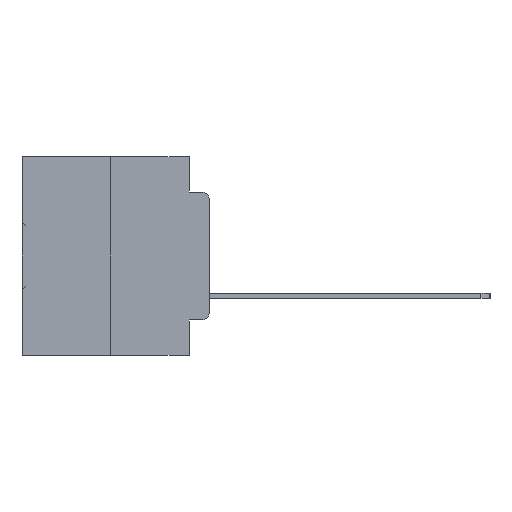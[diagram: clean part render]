
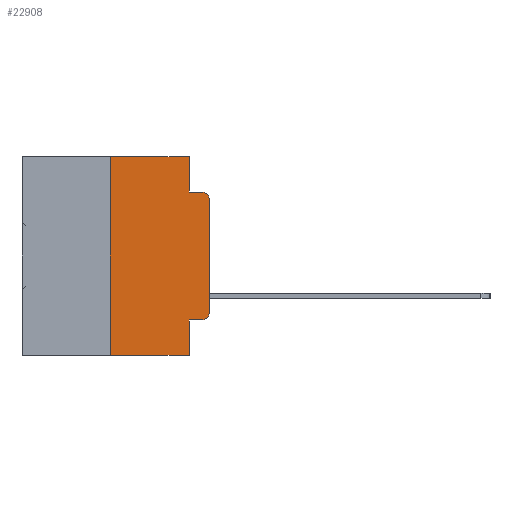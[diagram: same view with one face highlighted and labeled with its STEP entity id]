
A CAD part, left-side view. The second image highlights one B-rep face of the part: STEP entity #22908.
In plain terms, the highlighted planar face has unit normal (-1, 0, 0).
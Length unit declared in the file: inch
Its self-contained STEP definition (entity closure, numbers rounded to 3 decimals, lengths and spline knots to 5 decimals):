
#1056 = VECTOR ( 'NONE', #15404, 39.37008 ) ;
#1269 = CARTESIAN_POINT ( 'NONE',  ( 0., 0.051, -0.4115 ) ) ;
#1738 = ORIENTED_EDGE ( 'NONE', *, *, #35972, .T. ) ;
#2229 = ORIENTED_EDGE ( 'NONE', *, *, #19711, .F. ) ;
#2500 = DIRECTION ( 'NONE',  ( -1., 0., 0. ) ) ;
#3586 = CARTESIAN_POINT ( 'NONE',  ( 0., 0.25, -0.5 ) ) ;
#3743 = CARTESIAN_POINT ( 'NONE',  ( 0., 0.051, -0.4115 ) ) ;
#4054 = ORIENTED_EDGE ( 'NONE', *, *, #25440, .T. ) ;
#4241 = VECTOR ( 'NONE', #36297, 39.37008 ) ;
#4340 = VERTEX_POINT ( 'NONE', #30732 ) ;
#5243 = DIRECTION ( 'NONE',  ( 0., 0., -1. ) ) ;
#6064 = LINE ( 'NONE', #13987, #4241 ) ;
#6784 = CARTESIAN_POINT ( 'NONE',  ( 0., 0.02, -0.1085 ) ) ;
#7334 = VERTEX_POINT ( 'NONE', #12766 ) ;
#7928 = CARTESIAN_POINT ( 'NONE',  ( 0., 0.02, -0.4115 ) ) ;
#8266 = EDGE_LOOP ( 'NONE', ( #1738, #24762, #33824, #27350, #21691, #29962, #24350, #2229, #26063, #4054 ) ) ;
#8733 = LINE ( 'NONE', #10281, #33962 ) ;
#9096 = EDGE_CURVE ( 'NONE', #15135, #34101, #36450, .T. ) ;
#9732 = DIRECTION ( 'NONE',  ( 0., 0., -1. ) ) ;
#9747 = VECTOR ( 'NONE', #12873, 39.37008 ) ;
#9796 = VERTEX_POINT ( 'NONE', #31091 ) ;
#10281 = CARTESIAN_POINT ( 'NONE',  ( 0., 0.25, 0. ) ) ;
#10906 = DIRECTION ( 'NONE',  ( 1., 0., 0. ) ) ;
#11602 = DIRECTION ( 'NONE',  ( 0., -1., 0. ) ) ;
#11873 = CIRCLE ( 'NONE', #14674, 0.02 ) ;
#11953 = EDGE_CURVE ( 'NONE', #4340, #20574, #22420, .T. ) ;
#12243 = LINE ( 'NONE', #31392, #19895 ) ;
#12766 = CARTESIAN_POINT ( 'NONE',  ( 0., 0., -0.3915 ) ) ;
#12873 = DIRECTION ( 'NONE',  ( 0., -1., 0. ) ) ;
#13215 = DIRECTION ( 'NONE',  ( 0., 0., 1. ) ) ;
#13987 = CARTESIAN_POINT ( 'NONE',  ( 0., 0.473, 0. ) ) ;
#14126 = CARTESIAN_POINT ( 'NONE',  ( 0., 0.25, 0. ) ) ;
#14674 = AXIS2_PLACEMENT_3D ( 'NONE', #19851, #2500, #22746 ) ;
#15135 = VERTEX_POINT ( 'NONE', #1269 ) ;
#15404 = DIRECTION ( 'NONE',  ( 0., 0., 1. ) ) ;
#15636 = LINE ( 'NONE', #27138, #16526 ) ;
#16012 = DIRECTION ( 'NONE',  ( 0., 0., -1. ) ) ;
#16526 = VECTOR ( 'NONE', #16012, 39.37008 ) ;
#17277 = FACE_OUTER_BOUND ( 'NONE', #8266, .T. ) ;
#19446 = CARTESIAN_POINT ( 'NONE',  ( 0., 0.473, 0. ) ) ;
#19663 = EDGE_CURVE ( 'NONE', #9796, #20574, #32316, .T. ) ;
#19711 = EDGE_CURVE ( 'NONE', #15135, #25447, #15636, .T. ) ;
#19851 = CARTESIAN_POINT ( 'NONE',  ( 0., 0.02, -0.3915 ) ) ;
#19895 = VECTOR ( 'NONE', #11602, 39.37008 ) ;
#19955 = VECTOR ( 'NONE', #5243, 39.37008 ) ;
#20574 = VERTEX_POINT ( 'NONE', #32789 ) ;
#21527 = CARTESIAN_POINT ( 'NONE',  ( 0., 0.051, -0.0885 ) ) ;
#21691 = ORIENTED_EDGE ( 'NONE', *, *, #28326, .F. ) ;
#21794 = AXIS2_PLACEMENT_3D ( 'NONE', #6784, #26805, #9732 ) ;
#22075 = EDGE_CURVE ( 'NONE', #27479, #34710, #8733, .T. ) ;
#22420 = CIRCLE ( 'NONE', #21794, 0.02 ) ;
#22571 = CARTESIAN_POINT ( 'NONE',  ( 0., 0.051, 0. ) ) ;
#22730 = VERTEX_POINT ( 'NONE', #32839 ) ;
#22746 = DIRECTION ( 'NONE',  ( 0., 0., -1. ) ) ;
#22908 = ADVANCED_FACE ( 'NONE', ( #17277 ), #36146, .F. ) ;
#23246 = LINE ( 'NONE', #32216, #1056 ) ;
#23711 = EDGE_CURVE ( 'NONE', #27479, #25447, #12243, .T. ) ;
#24350 = ORIENTED_EDGE ( 'NONE', *, *, #23711, .T. ) ;
#24762 = ORIENTED_EDGE ( 'NONE', *, *, #11953, .T. ) ;
#25440 = EDGE_CURVE ( 'NONE', #34101, #7334, #11873, .T. ) ;
#25447 = VERTEX_POINT ( 'NONE', #30992 ) ;
#26063 = ORIENTED_EDGE ( 'NONE', *, *, #9096, .T. ) ;
#26800 = DIRECTION ( 'NONE',  ( 0., -1., 0. ) ) ;
#26805 = DIRECTION ( 'NONE',  ( -1., 0., 0. ) ) ;
#27138 = CARTESIAN_POINT ( 'NONE',  ( 0., 0.051, 0. ) ) ;
#27350 = ORIENTED_EDGE ( 'NONE', *, *, #30926, .F. ) ;
#27398 = LINE ( 'NONE', #22571, #19955 ) ;
#27479 = VERTEX_POINT ( 'NONE', #3586 ) ;
#28326 = EDGE_CURVE ( 'NONE', #34710, #22730, #6064, .T. ) ;
#28570 = AXIS2_PLACEMENT_3D ( 'NONE', #19446, #10906, #30699 ) ;
#29089 = VECTOR ( 'NONE', #26800, 39.37008 ) ;
#29962 = ORIENTED_EDGE ( 'NONE', *, *, #22075, .F. ) ;
#30699 = DIRECTION ( 'NONE',  ( 0., 0., -1. ) ) ;
#30732 = CARTESIAN_POINT ( 'NONE',  ( 0., 0., -0.1085 ) ) ;
#30926 = EDGE_CURVE ( 'NONE', #22730, #9796, #27398, .T. ) ;
#30992 = CARTESIAN_POINT ( 'NONE',  ( 0., 0.051, -0.5 ) ) ;
#31091 = CARTESIAN_POINT ( 'NONE',  ( 0., 0.051, -0.0885 ) ) ;
#31392 = CARTESIAN_POINT ( 'NONE',  ( 0., 0.473, -0.5 ) ) ;
#32216 = CARTESIAN_POINT ( 'NONE',  ( 0., 0., 0. ) ) ;
#32316 = LINE ( 'NONE', #21527, #9747 ) ;
#32789 = CARTESIAN_POINT ( 'NONE',  ( 0., 0.02, -0.0885 ) ) ;
#32839 = CARTESIAN_POINT ( 'NONE',  ( 0., 0.051, 0. ) ) ;
#33824 = ORIENTED_EDGE ( 'NONE', *, *, #19663, .F. ) ;
#33962 = VECTOR ( 'NONE', #13215, 39.37008 ) ;
#34101 = VERTEX_POINT ( 'NONE', #7928 ) ;
#34710 = VERTEX_POINT ( 'NONE', #14126 ) ;
#35972 = EDGE_CURVE ( 'NONE', #7334, #4340, #23246, .T. ) ;
#36146 = PLANE ( 'NONE',  #28570 ) ;
#36297 = DIRECTION ( 'NONE',  ( 0., -1., 0. ) ) ;
#36450 = LINE ( 'NONE', #3743, #29089 ) ;
